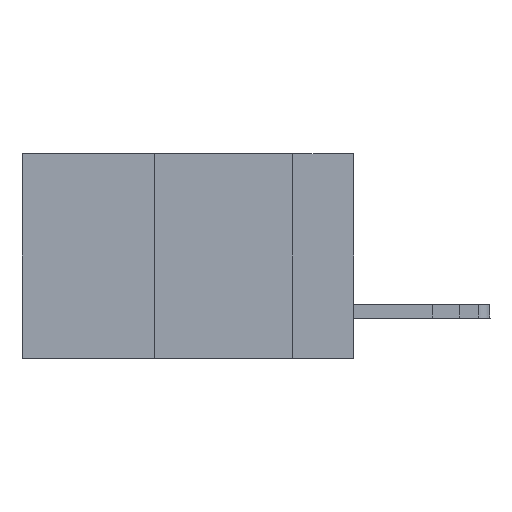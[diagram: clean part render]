
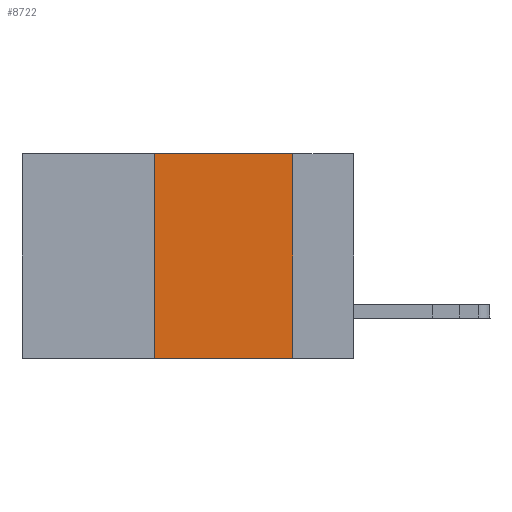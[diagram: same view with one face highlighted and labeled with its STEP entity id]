
A CAD part, left-side view. The second image highlights one B-rep face of the part: STEP entity #8722.
In plain terms, the highlighted planar face has unit normal (-1, 0, 0).
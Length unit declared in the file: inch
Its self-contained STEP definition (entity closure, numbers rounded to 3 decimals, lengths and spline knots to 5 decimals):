
#139 = EDGE_CURVE ( 'NONE', #1014, #556, #1004, .T. ) ;
#387 = ORIENTED_EDGE ( 'NONE', *, *, #13370, .F. ) ;
#556 = VERTEX_POINT ( 'NONE', #12207 ) ;
#1004 = LINE ( 'NONE', #10830, #1544 ) ;
#1014 = VERTEX_POINT ( 'NONE', #2270 ) ;
#1095 = LINE ( 'NONE', #8309, #2586 ) ;
#1179 = FACE_OUTER_BOUND ( 'NONE', #15376, .T. ) ;
#1193 = DIRECTION ( 'NONE',  ( 0., 0., -1. ) ) ;
#1544 = VECTOR ( 'NONE', #3821, 39.37008 ) ;
#1591 = VERTEX_POINT ( 'NONE', #5783 ) ;
#2270 = CARTESIAN_POINT ( 'NONE',  ( 0., 0.36, 0. ) ) ;
#2586 = VECTOR ( 'NONE', #1193, 39.37008 ) ;
#3634 = DIRECTION ( 'NONE',  ( 0., 0., -1. ) ) ;
#3821 = DIRECTION ( 'NONE',  ( 0., -1., 0. ) ) ;
#4054 = VERTEX_POINT ( 'NONE', #4974 ) ;
#4792 = LINE ( 'NONE', #15726, #12434 ) ;
#4974 = CARTESIAN_POINT ( 'NONE',  ( 0., 0.11, -0.37 ) ) ;
#5783 = CARTESIAN_POINT ( 'NONE',  ( 0., 0.36, -0.37 ) ) ;
#7932 = DIRECTION ( 'NONE',  ( 1., 0., 0. ) ) ;
#8199 = LINE ( 'NONE', #9594, #15987 ) ;
#8283 = DIRECTION ( 'NONE',  ( 0., -1., 0. ) ) ;
#8309 = CARTESIAN_POINT ( 'NONE',  ( 0., 0.11, 0. ) ) ;
#8722 = ADVANCED_FACE ( 'NONE', ( #1179 ), #10728, .F. ) ;
#9594 = CARTESIAN_POINT ( 'NONE',  ( 0., 0.6, -0.37 ) ) ;
#10447 = AXIS2_PLACEMENT_3D ( 'NONE', #10904, #7932, #3634 ) ;
#10728 = PLANE ( 'NONE',  #10447 ) ;
#10830 = CARTESIAN_POINT ( 'NONE',  ( 0., 0.6, 0. ) ) ;
#10904 = CARTESIAN_POINT ( 'NONE',  ( 0., 0.6, 0. ) ) ;
#11726 = EDGE_CURVE ( 'NONE', #1591, #4054, #8199, .T. ) ;
#12207 = CARTESIAN_POINT ( 'NONE',  ( 0., 0.11, 0. ) ) ;
#12434 = VECTOR ( 'NONE', #17422, 39.37008 ) ;
#13370 = EDGE_CURVE ( 'NONE', #1591, #1014, #4792, .T. ) ;
#14054 = EDGE_CURVE ( 'NONE', #556, #4054, #1095, .T. ) ;
#14467 = ORIENTED_EDGE ( 'NONE', *, *, #11726, .T. ) ;
#15376 = EDGE_LOOP ( 'NONE', ( #18125, #18509, #387, #14467 ) ) ;
#15726 = CARTESIAN_POINT ( 'NONE',  ( 0., 0.36, 0. ) ) ;
#15987 = VECTOR ( 'NONE', #8283, 39.37008 ) ;
#17422 = DIRECTION ( 'NONE',  ( 0., 0., 1. ) ) ;
#18125 = ORIENTED_EDGE ( 'NONE', *, *, #14054, .F. ) ;
#18509 = ORIENTED_EDGE ( 'NONE', *, *, #139, .F. ) ;
